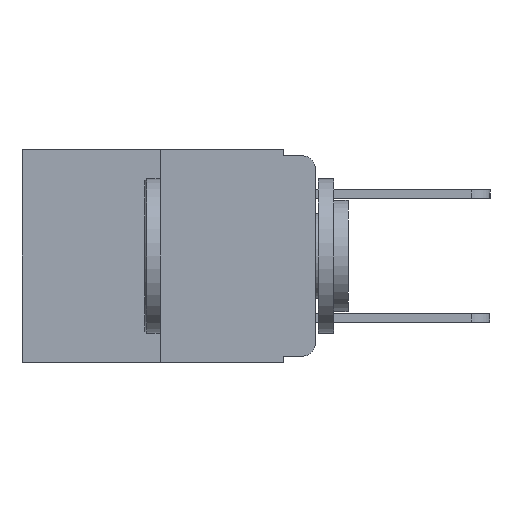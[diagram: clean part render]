
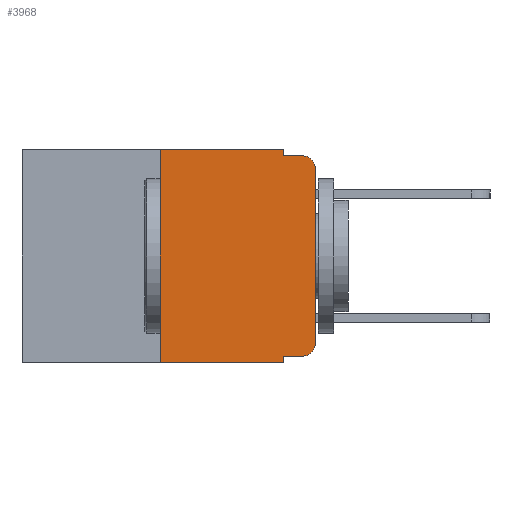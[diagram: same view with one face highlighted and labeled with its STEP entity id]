
A CAD part, left-side view. The second image highlights one B-rep face of the part: STEP entity #3968.
In plain terms, the highlighted planar face has unit normal (-1, 0, 0).
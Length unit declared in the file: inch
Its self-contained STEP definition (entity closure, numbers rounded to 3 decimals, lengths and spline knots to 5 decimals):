
#30 = VERTEX_POINT ( 'NONE', #2260 ) ;
#31 = VERTEX_POINT ( 'NONE', #2854 ) ;
#514 = VERTEX_POINT ( 'NONE', #7682 ) ;
#684 = VECTOR ( 'NONE', #7305, 39.37008 ) ;
#961 = LINE ( 'NONE', #5562, #5966 ) ;
#1288 = CARTESIAN_POINT ( 'NONE',  ( 0., 0.25, 0. ) ) ;
#1561 = DIRECTION ( 'NONE',  ( 0., 0., -1. ) ) ;
#1598 = CARTESIAN_POINT ( 'NONE',  ( 0., 0., -0.03 ) ) ;
#1634 = DIRECTION ( 'NONE',  ( 0., 0., 1. ) ) ;
#1701 = CARTESIAN_POINT ( 'NONE',  ( 0., 0.02, -0.03 ) ) ;
#1732 = VERTEX_POINT ( 'NONE', #3063 ) ;
#1834 = VECTOR ( 'NONE', #10117, 39.37008 ) ;
#2021 = DIRECTION ( 'NONE',  ( 0., 0., -1. ) ) ;
#2260 = CARTESIAN_POINT ( 'NONE',  ( 0., 0.02, -0.01 ) ) ;
#2274 = VERTEX_POINT ( 'NONE', #1598 ) ;
#2703 = DIRECTION ( 'NONE',  ( 0., 0., -1. ) ) ;
#2781 = VECTOR ( 'NONE', #6408, 39.37008 ) ;
#2854 = CARTESIAN_POINT ( 'NONE',  ( 0., 0., -0.313 ) ) ;
#3063 = CARTESIAN_POINT ( 'NONE',  ( 0., 0.25, -0.343 ) ) ;
#3082 = LINE ( 'NONE', #5415, #2781 ) ;
#3103 = CARTESIAN_POINT ( 'NONE',  ( 0., 0.051, -0.01 ) ) ;
#3240 = CIRCLE ( 'NONE', #10236, 0.02 ) ;
#3578 = DIRECTION ( 'NONE',  ( 0., -1., 0. ) ) ;
#3676 = LINE ( 'NONE', #6324, #684 ) ;
#3702 = AXIS2_PLACEMENT_3D ( 'NONE', #8803, #10474, #2021 ) ;
#3968 = ADVANCED_FACE ( 'NONE', ( #9513 ), #10960, .F. ) ;
#4153 = EDGE_CURVE ( 'NONE', #6048, #514, #4321, .T. ) ;
#4260 = ORIENTED_EDGE ( 'NONE', *, *, #7461, .T. ) ;
#4321 = LINE ( 'NONE', #7463, #6981 ) ;
#4342 = ORIENTED_EDGE ( 'NONE', *, *, #10470, .T. ) ;
#4420 = DIRECTION ( 'NONE',  ( 0., 0., 1. ) ) ;
#4454 = VERTEX_POINT ( 'NONE', #3103 ) ;
#4491 = VERTEX_POINT ( 'NONE', #5249 ) ;
#4603 = VERTEX_POINT ( 'NONE', #9518 ) ;
#4860 = CARTESIAN_POINT ( 'NONE',  ( 0., 0.051, -0.343 ) ) ;
#5030 = EDGE_LOOP ( 'NONE', ( #4342, #4260, #10539, #10081, #10840, #6601, #7108, #5510, #8783, #8928 ) ) ;
#5196 = CARTESIAN_POINT ( 'NONE',  ( 0., 0.051, -0.333 ) ) ;
#5211 = CARTESIAN_POINT ( 'NONE',  ( 0., 0.02, -0.313 ) ) ;
#5249 = CARTESIAN_POINT ( 'NONE',  ( 0., 0.051, -0.333 ) ) ;
#5403 = LINE ( 'NONE', #10007, #7671 ) ;
#5415 = CARTESIAN_POINT ( 'NONE',  ( 0., 0.051, 0. ) ) ;
#5493 = CARTESIAN_POINT ( 'NONE',  ( 0., 0.051, 0. ) ) ;
#5510 = ORIENTED_EDGE ( 'NONE', *, *, #7314, .F. ) ;
#5562 = CARTESIAN_POINT ( 'NONE',  ( 0., 0., 0. ) ) ;
#5950 = DIRECTION ( 'NONE',  ( 0., -1., 0. ) ) ;
#5966 = VECTOR ( 'NONE', #1634, 39.37008 ) ;
#6048 = VERTEX_POINT ( 'NONE', #1288 ) ;
#6324 = CARTESIAN_POINT ( 'NONE',  ( 0., 0.473, -0.343 ) ) ;
#6401 = AXIS2_PLACEMENT_3D ( 'NONE', #1701, #8487, #2703 ) ;
#6408 = DIRECTION ( 'NONE',  ( 0., 0., -1. ) ) ;
#6473 = CIRCLE ( 'NONE', #6401, 0.02 ) ;
#6601 = ORIENTED_EDGE ( 'NONE', *, *, #7351, .F. ) ;
#6981 = VECTOR ( 'NONE', #5950, 39.37008 ) ;
#7059 = EDGE_CURVE ( 'NONE', #4603, #31, #3240, .T. ) ;
#7096 = VECTOR ( 'NONE', #1561, 39.37008 ) ;
#7108 = ORIENTED_EDGE ( 'NONE', *, *, #7265, .T. ) ;
#7118 = EDGE_CURVE ( 'NONE', #4491, #4603, #10153, .T. ) ;
#7265 = EDGE_CURVE ( 'NONE', #1732, #8705, #3676, .T. ) ;
#7305 = DIRECTION ( 'NONE',  ( 0., -1., 0. ) ) ;
#7314 = EDGE_CURVE ( 'NONE', #4491, #8705, #3082, .T. ) ;
#7351 = EDGE_CURVE ( 'NONE', #1732, #6048, #5403, .T. ) ;
#7389 = EDGE_CURVE ( 'NONE', #514, #4454, #9467, .T. ) ;
#7396 = LINE ( 'NONE', #8383, #1834 ) ;
#7404 = EDGE_CURVE ( 'NONE', #4454, #30, #7396, .T. ) ;
#7461 = EDGE_CURVE ( 'NONE', #2274, #30, #6473, .T. ) ;
#7463 = CARTESIAN_POINT ( 'NONE',  ( 0., 0.473, 0. ) ) ;
#7671 = VECTOR ( 'NONE', #4420, 39.37008 ) ;
#7682 = CARTESIAN_POINT ( 'NONE',  ( 0., 0.051, 0. ) ) ;
#8131 = DIRECTION ( 'NONE',  ( 0., 0., -1. ) ) ;
#8383 = CARTESIAN_POINT ( 'NONE',  ( 0., 0.051, -0.01 ) ) ;
#8487 = DIRECTION ( 'NONE',  ( -1., 0., 0. ) ) ;
#8705 = VERTEX_POINT ( 'NONE', #4860 ) ;
#8783 = ORIENTED_EDGE ( 'NONE', *, *, #7118, .T. ) ;
#8803 = CARTESIAN_POINT ( 'NONE',  ( 0., 0.473, 0. ) ) ;
#8928 = ORIENTED_EDGE ( 'NONE', *, *, #7059, .T. ) ;
#9467 = LINE ( 'NONE', #5493, #7096 ) ;
#9513 = FACE_OUTER_BOUND ( 'NONE', #5030, .T. ) ;
#9518 = CARTESIAN_POINT ( 'NONE',  ( 0., 0.02, -0.333 ) ) ;
#9891 = VECTOR ( 'NONE', #3578, 39.37008 ) ;
#10007 = CARTESIAN_POINT ( 'NONE',  ( 0., 0.25, 0. ) ) ;
#10081 = ORIENTED_EDGE ( 'NONE', *, *, #7389, .F. ) ;
#10117 = DIRECTION ( 'NONE',  ( 0., -1., 0. ) ) ;
#10153 = LINE ( 'NONE', #5196, #9891 ) ;
#10236 = AXIS2_PLACEMENT_3D ( 'NONE', #5211, #10548, #8131 ) ;
#10470 = EDGE_CURVE ( 'NONE', #31, #2274, #961, .T. ) ;
#10474 = DIRECTION ( 'NONE',  ( 1., 0., 0. ) ) ;
#10539 = ORIENTED_EDGE ( 'NONE', *, *, #7404, .F. ) ;
#10548 = DIRECTION ( 'NONE',  ( -1., 0., 0. ) ) ;
#10840 = ORIENTED_EDGE ( 'NONE', *, *, #4153, .F. ) ;
#10960 = PLANE ( 'NONE',  #3702 ) ;
